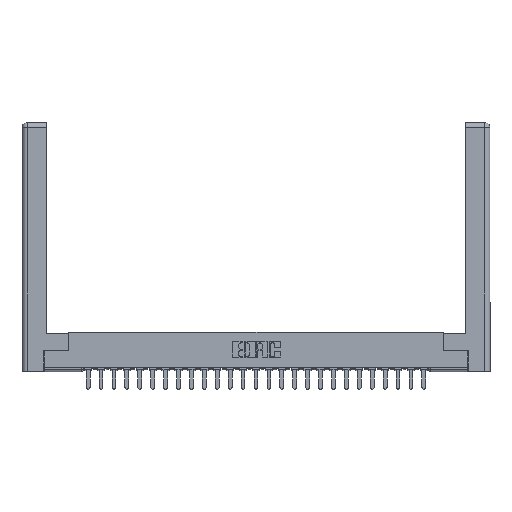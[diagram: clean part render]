
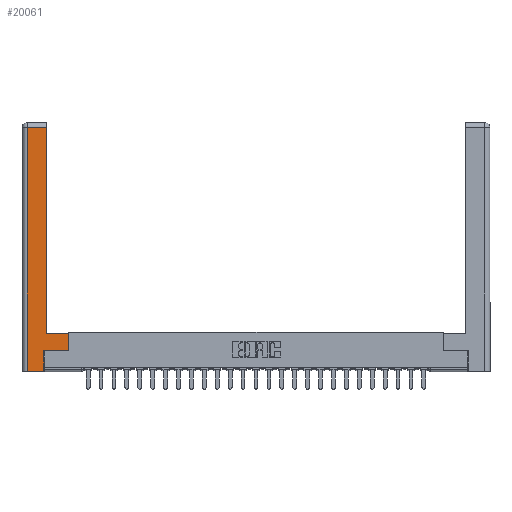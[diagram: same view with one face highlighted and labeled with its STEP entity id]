
A CAD part, top view. The second image highlights one B-rep face of the part: STEP entity #20061.
In plain terms, the highlighted planar face has unit normal (0, 0, 1).
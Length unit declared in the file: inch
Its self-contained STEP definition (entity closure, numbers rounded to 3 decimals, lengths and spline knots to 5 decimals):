
#252 = VERTEX_POINT ( 'NONE', #23490 ) ;
#400 = VERTEX_POINT ( 'NONE', #17388 ) ;
#537 = ORIENTED_EDGE ( 'NONE', *, *, #25421, .T. ) ;
#1150 = EDGE_CURVE ( 'NONE', #24989, #23032, #22553, .T. ) ;
#1707 = VECTOR ( 'NONE', #18997, 39.37008 ) ;
#3125 = AXIS2_PLACEMENT_3D ( 'NONE', #21943, #21847, #4500 ) ;
#4500 = DIRECTION ( 'NONE',  ( -1., 0., 0. ) ) ;
#4589 = PLANE ( 'NONE',  #3125 ) ;
#4624 = ORIENTED_EDGE ( 'NONE', *, *, #1150, .T. ) ;
#6828 = ORIENTED_EDGE ( 'NONE', *, *, #22926, .T. ) ;
#7451 = VERTEX_POINT ( 'NONE', #12887 ) ;
#7523 = EDGE_CURVE ( 'NONE', #27720, #12454, #10467, .T. ) ;
#7885 = LINE ( 'NONE', #16727, #11244 ) ;
#8368 = CARTESIAN_POINT ( 'NONE',  ( 0.265, 0., 0. ) ) ;
#9284 = EDGE_CURVE ( 'NONE', #23032, #15577, #11012, .T. ) ;
#9781 = LINE ( 'NONE', #10229, #21349 ) ;
#10146 = DIRECTION ( 'NONE',  ( 0., 1., 0. ) ) ;
#10229 = CARTESIAN_POINT ( 'NONE',  ( 0.565, 0.245, 0. ) ) ;
#10467 = LINE ( 'NONE', #10892, #25453 ) ;
#10892 = CARTESIAN_POINT ( 'NONE',  ( 0.0615, 0., 0. ) ) ;
#11012 = LINE ( 'NONE', #25582, #23942 ) ;
#11244 = VECTOR ( 'NONE', #23475, 39.37008 ) ;
#11491 = CARTESIAN_POINT ( 'NONE',  ( 0.295, 0.45, 0. ) ) ;
#12454 = VERTEX_POINT ( 'NONE', #18119 ) ;
#12887 = CARTESIAN_POINT ( 'NONE',  ( 0.265, 0., 0. ) ) ;
#13263 = DIRECTION ( 'NONE',  ( 0., -1., 0. ) ) ;
#13590 = CARTESIAN_POINT ( 'NONE',  ( 0.565, 0.45, 0. ) ) ;
#14213 = CARTESIAN_POINT ( 'NONE',  ( 0.295, 3., 0. ) ) ;
#14400 = DIRECTION ( 'NONE',  ( 0., 1., 0. ) ) ;
#15202 = EDGE_LOOP ( 'NONE', ( #25937, #6828, #25478, #25664, #537, #21222, #4624, #16963 ) ) ;
#15577 = VERTEX_POINT ( 'NONE', #11491 ) ;
#16469 = CARTESIAN_POINT ( 'NONE',  ( 0.265, 0.245, 0. ) ) ;
#16727 = CARTESIAN_POINT ( 'NONE',  ( 0.0615, 2.94, 0. ) ) ;
#16963 = ORIENTED_EDGE ( 'NONE', *, *, #9284, .T. ) ;
#17388 = CARTESIAN_POINT ( 'NONE',  ( 0.295, 2.94, 0. ) ) ;
#17424 = VECTOR ( 'NONE', #26255, 39.37008 ) ;
#18119 = CARTESIAN_POINT ( 'NONE',  ( 0.0615, 0., 0. ) ) ;
#18765 = VECTOR ( 'NONE', #14400, 39.37008 ) ;
#18997 = DIRECTION ( 'NONE',  ( 1., 0., 0. ) ) ;
#19732 = LINE ( 'NONE', #16469, #27956 ) ;
#20061 = ADVANCED_FACE ( 'NONE', ( #26140 ), #4589, .F. ) ;
#20442 = EDGE_CURVE ( 'NONE', #252, #24989, #9781, .T. ) ;
#20926 = DIRECTION ( 'NONE',  ( -1., 0., 0. ) ) ;
#21222 = ORIENTED_EDGE ( 'NONE', *, *, #20442, .T. ) ;
#21349 = VECTOR ( 'NONE', #27784, 39.37008 ) ;
#21847 = DIRECTION ( 'NONE',  ( 0., 0., -1. ) ) ;
#21943 = CARTESIAN_POINT ( 'NONE',  ( 0., 0., 0. ) ) ;
#22553 = LINE ( 'NONE', #13590, #17424 ) ;
#22926 = EDGE_CURVE ( 'NONE', #400, #27720, #7885, .T. ) ;
#22966 = EDGE_CURVE ( 'NONE', #12454, #7451, #27366, .T. ) ;
#23032 = VERTEX_POINT ( 'NONE', #23760 ) ;
#23226 = LINE ( 'NONE', #14213, #18765 ) ;
#23475 = DIRECTION ( 'NONE',  ( -1., 0., 0. ) ) ;
#23490 = CARTESIAN_POINT ( 'NONE',  ( 0.265, 0.245, 0. ) ) ;
#23760 = CARTESIAN_POINT ( 'NONE',  ( 0.565, 0.45, 0. ) ) ;
#23805 = CARTESIAN_POINT ( 'NONE',  ( 0.0615, 2.94, 0. ) ) ;
#23942 = VECTOR ( 'NONE', #20926, 39.37008 ) ;
#24020 = EDGE_CURVE ( 'NONE', #15577, #400, #23226, .T. ) ;
#24989 = VERTEX_POINT ( 'NONE', #26055 ) ;
#25421 = EDGE_CURVE ( 'NONE', #7451, #252, #19732, .T. ) ;
#25453 = VECTOR ( 'NONE', #13263, 39.37008 ) ;
#25478 = ORIENTED_EDGE ( 'NONE', *, *, #7523, .T. ) ;
#25582 = CARTESIAN_POINT ( 'NONE',  ( 0.295, 0.45, 0. ) ) ;
#25664 = ORIENTED_EDGE ( 'NONE', *, *, #22966, .T. ) ;
#25937 = ORIENTED_EDGE ( 'NONE', *, *, #24020, .T. ) ;
#26055 = CARTESIAN_POINT ( 'NONE',  ( 0.565, 0.245, 0. ) ) ;
#26140 = FACE_OUTER_BOUND ( 'NONE', #15202, .T. ) ;
#26255 = DIRECTION ( 'NONE',  ( 0., 1., 0. ) ) ;
#27366 = LINE ( 'NONE', #8368, #1707 ) ;
#27720 = VERTEX_POINT ( 'NONE', #23805 ) ;
#27784 = DIRECTION ( 'NONE',  ( 1., 0., 0. ) ) ;
#27956 = VECTOR ( 'NONE', #10146, 39.37008 ) ;
